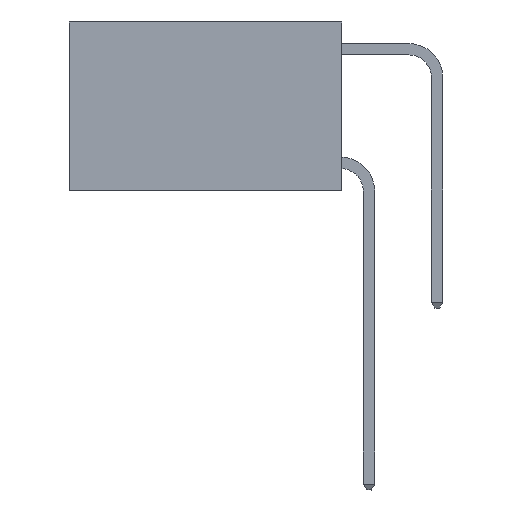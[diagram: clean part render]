
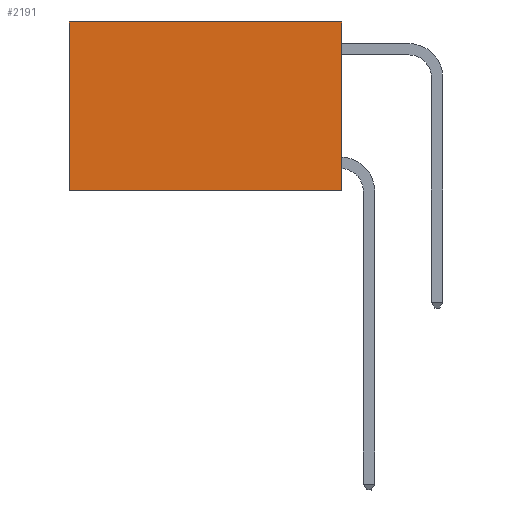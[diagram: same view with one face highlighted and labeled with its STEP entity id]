
A CAD part, left-side view. The second image highlights one B-rep face of the part: STEP entity #2191.
In plain terms, the highlighted planar face has unit normal (-1, 0, 0).
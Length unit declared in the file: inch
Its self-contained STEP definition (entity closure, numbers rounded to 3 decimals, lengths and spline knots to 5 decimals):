
#111 = AXIS2_PLACEMENT_3D ( 'NONE', #1075, #24101, #7082 ) ;
#166 = CARTESIAN_POINT ( 'NONE',  ( 0.2625, 0.6, 0. ) ) ;
#908 = VERTEX_POINT ( 'NONE', #22682 ) ;
#1075 = CARTESIAN_POINT ( 'NONE',  ( 0.2625, 0., 0. ) ) ;
#1365 = EDGE_CURVE ( 'NONE', #908, #13103, #16029, .T. ) ;
#2191 = ADVANCED_FACE ( 'NONE', ( #20329 ), #24450, .F. ) ;
#4703 = CARTESIAN_POINT ( 'NONE',  ( 0.2625, 0., 0. ) ) ;
#5426 = CARTESIAN_POINT ( 'NONE',  ( 0.2625, 0.6, -0.37 ) ) ;
#6212 = CARTESIAN_POINT ( 'NONE',  ( 0.2625, 0., -0.37 ) ) ;
#6326 = LINE ( 'NONE', #6212, #19352 ) ;
#7082 = DIRECTION ( 'NONE',  ( 0., 0., -1. ) ) ;
#7822 = DIRECTION ( 'NONE',  ( 0., 0., -1. ) ) ;
#8776 = VERTEX_POINT ( 'NONE', #12436 ) ;
#9307 = ORIENTED_EDGE ( 'NONE', *, *, #14200, .F. ) ;
#10417 = VECTOR ( 'NONE', #23573, 39.37008 ) ;
#10501 = CARTESIAN_POINT ( 'NONE',  ( 0.2625, 0., 0. ) ) ;
#11516 = DIRECTION ( 'NONE',  ( 0., 1., 0. ) ) ;
#12436 = CARTESIAN_POINT ( 'NONE',  ( 0.2625, 0., -0.37 ) ) ;
#13103 = VERTEX_POINT ( 'NONE', #5426 ) ;
#13351 = VECTOR ( 'NONE', #13992, 39.37008 ) ;
#13650 = EDGE_LOOP ( 'NONE', ( #22922, #22981, #9307, #19875 ) ) ;
#13739 = VECTOR ( 'NONE', #7822, 39.37008 ) ;
#13992 = DIRECTION ( 'NONE',  ( 0., 0., -1. ) ) ;
#14175 = EDGE_CURVE ( 'NONE', #8776, #13103, #6326, .T. ) ;
#14200 = EDGE_CURVE ( 'NONE', #17559, #8776, #17319, .T. ) ;
#14402 = LINE ( 'NONE', #4703, #10417 ) ;
#16029 = LINE ( 'NONE', #166, #13351 ) ;
#17319 = LINE ( 'NONE', #17442, #13739 ) ;
#17442 = CARTESIAN_POINT ( 'NONE',  ( 0.2625, 0., 0. ) ) ;
#17559 = VERTEX_POINT ( 'NONE', #10501 ) ;
#19352 = VECTOR ( 'NONE', #11516, 39.37008 ) ;
#19875 = ORIENTED_EDGE ( 'NONE', *, *, #22709, .T. ) ;
#20329 = FACE_OUTER_BOUND ( 'NONE', #13650, .T. ) ;
#22682 = CARTESIAN_POINT ( 'NONE',  ( 0.2625, 0.6, 0. ) ) ;
#22709 = EDGE_CURVE ( 'NONE', #17559, #908, #14402, .T. ) ;
#22922 = ORIENTED_EDGE ( 'NONE', *, *, #1365, .T. ) ;
#22981 = ORIENTED_EDGE ( 'NONE', *, *, #14175, .F. ) ;
#23573 = DIRECTION ( 'NONE',  ( 0., 1., 0. ) ) ;
#24101 = DIRECTION ( 'NONE',  ( 1., 0., 0. ) ) ;
#24450 = PLANE ( 'NONE',  #111 ) ;
